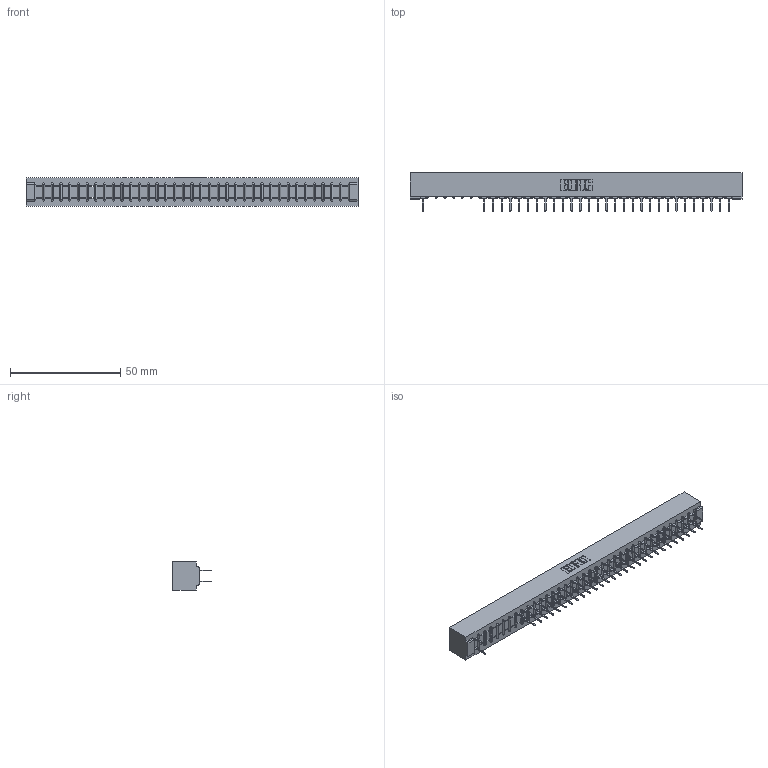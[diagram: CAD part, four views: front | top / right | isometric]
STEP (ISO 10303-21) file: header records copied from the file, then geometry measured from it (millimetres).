
FILE_DESCRIPTION (( 'STEP AP203' ), '1' );
FILE_NAME ('307-072-524-201.STEP', '2018-08-06T13:51:06', ( '' ), ( '' ), 'SwSTEP 2.0', 'SolidWorks 2016', '' );
FILE_SCHEMA (( 'CONFIG_CONTROL_DESIGN' ));
Length unit declared in the file: inch
Products named in the file (3): 307-072-524-201; 307 Part_No Mounting Lugs; 307-290-001_524
Assembly tree (60 placements, depth 2):
  307-072-524-201
    307 Part_No Mounting Lugs
    307-290-001_524  x59
Bounding box: 150.52 x 17.42 x 12.7 mm (x, y, z)
Volume: 16323.7 mm3; surface area: 18859.9 mm2
Topology: 60 solids, 60 shells, 2991 faces, 8385 edges, 5410 vertices
Faces by surface type: plane 1973, cylinder 944, sphere 74
Entity records: 32028 total; most frequent: CARTESIAN_POINT 5291, ORIENTED_EDGE 5254, DIRECTION 5171, EDGE_CURVE 2627, VECTOR 2015, LINE 2015, VERTEX_POINT 1698, AXIS2_PLACEMENT_3D 1578
